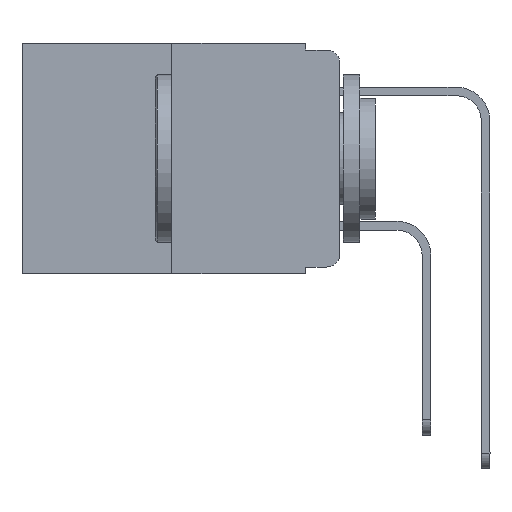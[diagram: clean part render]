
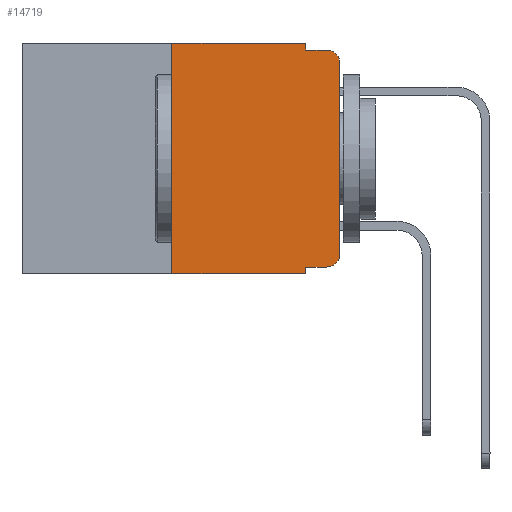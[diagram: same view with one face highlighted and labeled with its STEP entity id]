
A CAD part, left-side view. The second image highlights one B-rep face of the part: STEP entity #14719.
In plain terms, the highlighted planar face has unit normal (-1, 0, 0).
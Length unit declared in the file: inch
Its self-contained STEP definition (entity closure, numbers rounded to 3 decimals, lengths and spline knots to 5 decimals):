
#121 = DIRECTION ( 'NONE',  ( 0., 0., -1. ) ) ;
#719 = CARTESIAN_POINT ( 'NONE',  ( 0., 0.051, 0. ) ) ;
#792 = VECTOR ( 'NONE', #2739, 39.37008 ) ;
#1261 = LINE ( 'NONE', #4753, #6695 ) ;
#1414 = ORIENTED_EDGE ( 'NONE', *, *, #10435, .T. ) ;
#1441 = CARTESIAN_POINT ( 'NONE',  ( 0., 0.051, -0.01 ) ) ;
#1734 = VERTEX_POINT ( 'NONE', #15010 ) ;
#1951 = LINE ( 'NONE', #16070, #15782 ) ;
#2041 = EDGE_CURVE ( 'NONE', #1734, #4889, #10826, .T. ) ;
#2166 = EDGE_CURVE ( 'NONE', #4889, #10478, #13098, .T. ) ;
#2276 = DIRECTION ( 'NONE',  ( 0., -1., 0. ) ) ;
#2676 = VERTEX_POINT ( 'NONE', #12267 ) ;
#2701 = AXIS2_PLACEMENT_3D ( 'NONE', #9366, #9451, #8297 ) ;
#2739 = DIRECTION ( 'NONE',  ( 0., -1., 0. ) ) ;
#3307 = ORIENTED_EDGE ( 'NONE', *, *, #10227, .F. ) ;
#3374 = VERTEX_POINT ( 'NONE', #11073 ) ;
#3530 = CARTESIAN_POINT ( 'NONE',  ( 0., 0.051, -0.333 ) ) ;
#3993 = LINE ( 'NONE', #6364, #15185 ) ;
#4753 = CARTESIAN_POINT ( 'NONE',  ( 0., 0.051, -0.333 ) ) ;
#4775 = CARTESIAN_POINT ( 'NONE',  ( 0., 0., 0. ) ) ;
#4798 = CARTESIAN_POINT ( 'NONE',  ( 0., 0.051, -0.01 ) ) ;
#4853 = DIRECTION ( 'NONE',  ( 0., 0., 1. ) ) ;
#4889 = VERTEX_POINT ( 'NONE', #4798 ) ;
#5025 = AXIS2_PLACEMENT_3D ( 'NONE', #9974, #5068, #11290 ) ;
#5068 = DIRECTION ( 'NONE',  ( 1., 0., 0. ) ) ;
#5249 = VERTEX_POINT ( 'NONE', #8264 ) ;
#6013 = EDGE_LOOP ( 'NONE', ( #13435, #9538, #6734, #10576, #3307, #10918, #6805, #9309, #9061, #1414 ) ) ;
#6181 = CARTESIAN_POINT ( 'NONE',  ( 0., 0.02, -0.01 ) ) ;
#6233 = EDGE_CURVE ( 'NONE', #9364, #9705, #1261, .T. ) ;
#6364 = CARTESIAN_POINT ( 'NONE',  ( 0., 0.473, -0.343 ) ) ;
#6516 = CARTESIAN_POINT ( 'NONE',  ( 0., 0., -0.03 ) ) ;
#6695 = VECTOR ( 'NONE', #11205, 39.37008 ) ;
#6734 = ORIENTED_EDGE ( 'NONE', *, *, #2166, .F. ) ;
#6805 = ORIENTED_EDGE ( 'NONE', *, *, #14077, .T. ) ;
#7375 = PLANE ( 'NONE',  #5025 ) ;
#7556 = VECTOR ( 'NONE', #121, 39.37008 ) ;
#7663 = DIRECTION ( 'NONE',  ( 0., -1., 0. ) ) ;
#7843 = VECTOR ( 'NONE', #9201, 39.37008 ) ;
#8264 = CARTESIAN_POINT ( 'NONE',  ( 0., 0.25, -0.343 ) ) ;
#8297 = DIRECTION ( 'NONE',  ( 0., 0., -1. ) ) ;
#8988 = VECTOR ( 'NONE', #15905, 39.37008 ) ;
#9061 = ORIENTED_EDGE ( 'NONE', *, *, #6233, .T. ) ;
#9201 = DIRECTION ( 'NONE',  ( 0., 0., 1. ) ) ;
#9309 = ORIENTED_EDGE ( 'NONE', *, *, #12060, .F. ) ;
#9364 = VERTEX_POINT ( 'NONE', #3530 ) ;
#9366 = CARTESIAN_POINT ( 'NONE',  ( 0., 0.02, -0.03 ) ) ;
#9441 = CARTESIAN_POINT ( 'NONE',  ( 0., 0.25, 0. ) ) ;
#9451 = DIRECTION ( 'NONE',  ( -1., 0., 0. ) ) ;
#9538 = ORIENTED_EDGE ( 'NONE', *, *, #15579, .T. ) ;
#9705 = VERTEX_POINT ( 'NONE', #10421 ) ;
#9974 = CARTESIAN_POINT ( 'NONE',  ( 0., 0.473, 0. ) ) ;
#9989 = CARTESIAN_POINT ( 'NONE',  ( 0., 0.051, 0. ) ) ;
#9999 = CIRCLE ( 'NONE', #2701, 0.02 ) ;
#10227 = EDGE_CURVE ( 'NONE', #2676, #1734, #1951, .T. ) ;
#10421 = CARTESIAN_POINT ( 'NONE',  ( 0., 0.02, -0.333 ) ) ;
#10435 = EDGE_CURVE ( 'NONE', #9705, #3374, #12740, .T. ) ;
#10436 = CARTESIAN_POINT ( 'NONE',  ( 0., 0.051, -0.343 ) ) ;
#10478 = VERTEX_POINT ( 'NONE', #6181 ) ;
#10576 = ORIENTED_EDGE ( 'NONE', *, *, #2041, .F. ) ;
#10826 = LINE ( 'NONE', #719, #8988 ) ;
#10918 = ORIENTED_EDGE ( 'NONE', *, *, #12619, .F. ) ;
#11073 = CARTESIAN_POINT ( 'NONE',  ( 0., 0., -0.313 ) ) ;
#11205 = DIRECTION ( 'NONE',  ( 0., -1., 0. ) ) ;
#11290 = DIRECTION ( 'NONE',  ( 0., 0., -1. ) ) ;
#11326 = VERTEX_POINT ( 'NONE', #10436 ) ;
#11371 = DIRECTION ( 'NONE',  ( -1., 0., 0. ) ) ;
#11532 = CARTESIAN_POINT ( 'NONE',  ( 0., 0.02, -0.313 ) ) ;
#12060 = EDGE_CURVE ( 'NONE', #9364, #11326, #12448, .T. ) ;
#12216 = AXIS2_PLACEMENT_3D ( 'NONE', #11532, #11371, #14155 ) ;
#12267 = CARTESIAN_POINT ( 'NONE',  ( 0., 0.25, 0. ) ) ;
#12448 = LINE ( 'NONE', #9989, #7556 ) ;
#12523 = VERTEX_POINT ( 'NONE', #6516 ) ;
#12619 = EDGE_CURVE ( 'NONE', #5249, #2676, #13288, .T. ) ;
#12740 = CIRCLE ( 'NONE', #12216, 0.02 ) ;
#13098 = LINE ( 'NONE', #1441, #792 ) ;
#13288 = LINE ( 'NONE', #9441, #7843 ) ;
#13435 = ORIENTED_EDGE ( 'NONE', *, *, #16046, .T. ) ;
#13440 = LINE ( 'NONE', #4775, #15237 ) ;
#14077 = EDGE_CURVE ( 'NONE', #5249, #11326, #3993, .T. ) ;
#14155 = DIRECTION ( 'NONE',  ( 0., 0., -1. ) ) ;
#14719 = ADVANCED_FACE ( 'NONE', ( #14970 ), #7375, .F. ) ;
#14970 = FACE_OUTER_BOUND ( 'NONE', #6013, .T. ) ;
#15010 = CARTESIAN_POINT ( 'NONE',  ( 0., 0.051, 0. ) ) ;
#15185 = VECTOR ( 'NONE', #7663, 39.37008 ) ;
#15237 = VECTOR ( 'NONE', #4853, 39.37008 ) ;
#15579 = EDGE_CURVE ( 'NONE', #12523, #10478, #9999, .T. ) ;
#15782 = VECTOR ( 'NONE', #2276, 39.37008 ) ;
#15905 = DIRECTION ( 'NONE',  ( 0., 0., -1. ) ) ;
#16046 = EDGE_CURVE ( 'NONE', #3374, #12523, #13440, .T. ) ;
#16070 = CARTESIAN_POINT ( 'NONE',  ( 0., 0.473, 0. ) ) ;
